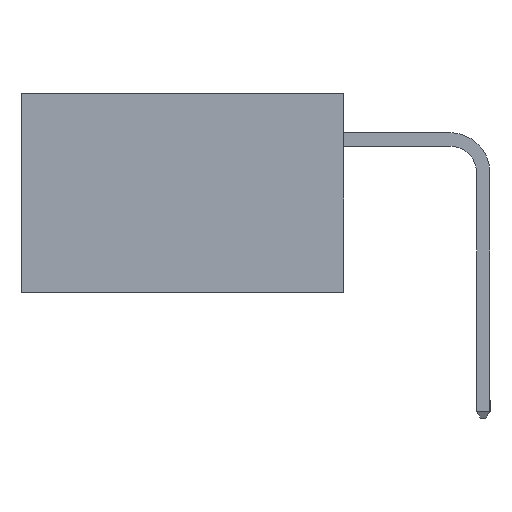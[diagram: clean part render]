
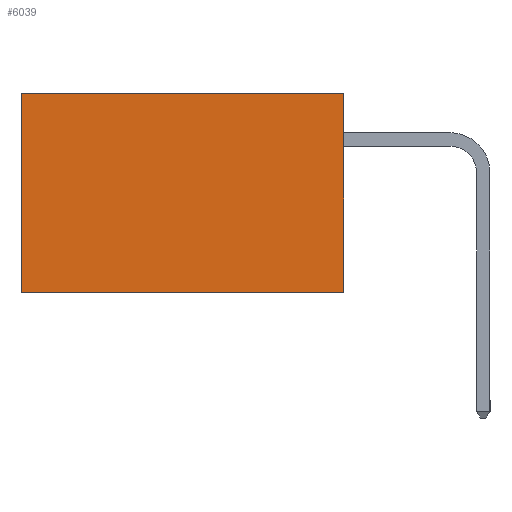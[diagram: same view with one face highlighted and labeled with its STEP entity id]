
A CAD part, left-side view. The second image highlights one B-rep face of the part: STEP entity #6039.
In plain terms, the highlighted planar face has unit normal (-1, 0, 0).
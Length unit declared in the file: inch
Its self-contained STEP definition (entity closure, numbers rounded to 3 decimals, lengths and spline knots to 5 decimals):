
#218 = VERTEX_POINT ( 'NONE', #2688 ) ;
#401 = LINE ( 'NONE', #11753, #10629 ) ;
#585 = FACE_OUTER_BOUND ( 'NONE', #3113, .T. ) ;
#741 = CARTESIAN_POINT ( 'NONE',  ( 0.2615, 0., -0.37 ) ) ;
#1711 = DIRECTION ( 'NONE',  ( 0., 0., -1. ) ) ;
#1742 = DIRECTION ( 'NONE',  ( 0., 1., 0. ) ) ;
#1857 = LINE ( 'NONE', #9820, #11777 ) ;
#2023 = AXIS2_PLACEMENT_3D ( 'NONE', #741, #7485, #1711 ) ;
#2118 = DIRECTION ( 'NONE',  ( 0., 0., -1. ) ) ;
#2137 = ORIENTED_EDGE ( 'NONE', *, *, #5047, .T. ) ;
#2688 = CARTESIAN_POINT ( 'NONE',  ( 0.2615, 0., 0. ) ) ;
#2786 = VERTEX_POINT ( 'NONE', #5196 ) ;
#3092 = DIRECTION ( 'NONE',  ( 0., 0., -1. ) ) ;
#3113 = EDGE_LOOP ( 'NONE', ( #2137, #12340, #10584, #5169 ) ) ;
#3272 = CARTESIAN_POINT ( 'NONE',  ( 0.2615, 0., 0. ) ) ;
#3615 = PLANE ( 'NONE',  #2023 ) ;
#4242 = DIRECTION ( 'NONE',  ( 0., 1., 0. ) ) ;
#4754 = CARTESIAN_POINT ( 'NONE',  ( 0.2615, 0.6, 0. ) ) ;
#5047 = EDGE_CURVE ( 'NONE', #6136, #2786, #1857, .T. ) ;
#5082 = VERTEX_POINT ( 'NONE', #8061 ) ;
#5169 = ORIENTED_EDGE ( 'NONE', *, *, #6655, .T. ) ;
#5196 = CARTESIAN_POINT ( 'NONE',  ( 0.2615, 0.6, -0.37 ) ) ;
#6039 = ADVANCED_FACE ( 'NONE', ( #585 ), #3615, .F. ) ;
#6136 = VERTEX_POINT ( 'NONE', #4754 ) ;
#6655 = EDGE_CURVE ( 'NONE', #218, #6136, #9325, .T. ) ;
#7180 = EDGE_CURVE ( 'NONE', #218, #5082, #401, .T. ) ;
#7485 = DIRECTION ( 'NONE',  ( 1., 0., 0. ) ) ;
#7489 = EDGE_CURVE ( 'NONE', #5082, #2786, #9760, .T. ) ;
#7828 = VECTOR ( 'NONE', #1742, 39.37008 ) ;
#8061 = CARTESIAN_POINT ( 'NONE',  ( 0.2615, 0., -0.37 ) ) ;
#8498 = CARTESIAN_POINT ( 'NONE',  ( 0.2615, 0., -0.37 ) ) ;
#9325 = LINE ( 'NONE', #3272, #11254 ) ;
#9760 = LINE ( 'NONE', #8498, #7828 ) ;
#9820 = CARTESIAN_POINT ( 'NONE',  ( 0.2615, 0.6, -0.37 ) ) ;
#10584 = ORIENTED_EDGE ( 'NONE', *, *, #7180, .F. ) ;
#10629 = VECTOR ( 'NONE', #2118, 39.37008 ) ;
#11254 = VECTOR ( 'NONE', #4242, 39.37008 ) ;
#11753 = CARTESIAN_POINT ( 'NONE',  ( 0.2615, 0., -0.37 ) ) ;
#11777 = VECTOR ( 'NONE', #3092, 39.37008 ) ;
#12340 = ORIENTED_EDGE ( 'NONE', *, *, #7489, .F. ) ;
